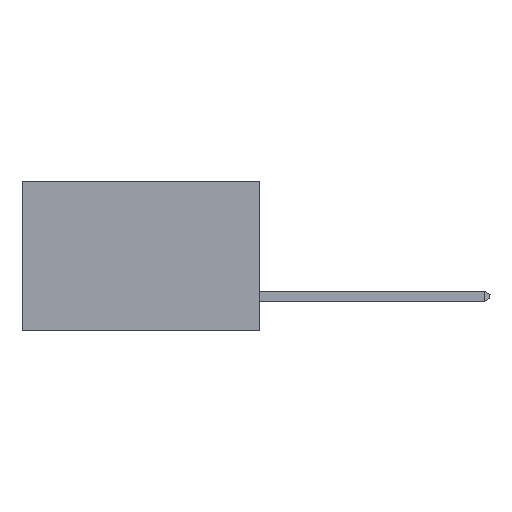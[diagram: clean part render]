
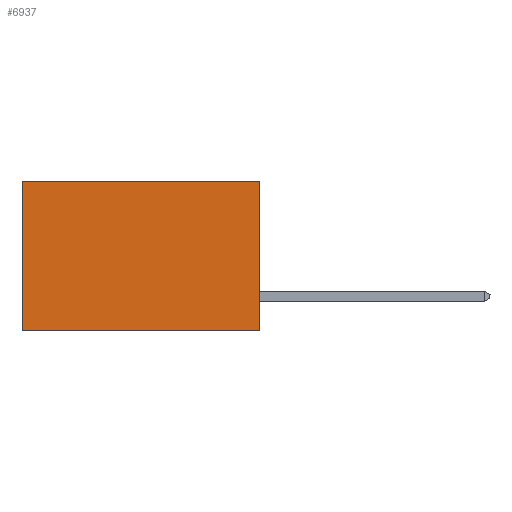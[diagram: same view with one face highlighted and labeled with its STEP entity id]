
A CAD part, left-side view. The second image highlights one B-rep face of the part: STEP entity #6937.
In plain terms, the highlighted planar face has unit normal (-1, 0, 0).
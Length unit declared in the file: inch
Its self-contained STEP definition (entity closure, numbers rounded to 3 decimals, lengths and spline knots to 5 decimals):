
#18 = FACE_OUTER_BOUND ( 'NONE', #20292, .T. ) ;
#437 = CARTESIAN_POINT ( 'NONE',  ( 0.277, 0., -0.37 ) ) ;
#490 = LINE ( 'NONE', #5966, #13847 ) ;
#847 = ORIENTED_EDGE ( 'NONE', *, *, #16687, .F. ) ;
#1221 = ORIENTED_EDGE ( 'NONE', *, *, #8267, .T. ) ;
#3124 = ORIENTED_EDGE ( 'NONE', *, *, #20080, .T. ) ;
#3379 = DIRECTION ( 'NONE',  ( 1., 0., 0. ) ) ;
#3512 = CARTESIAN_POINT ( 'NONE',  ( 0.277, 0., -0.37 ) ) ;
#4038 = AXIS2_PLACEMENT_3D ( 'NONE', #437, #3379, #16600 ) ;
#5423 = VERTEX_POINT ( 'NONE', #14707 ) ;
#5966 = CARTESIAN_POINT ( 'NONE',  ( 0.277, 0.59, -0.37 ) ) ;
#6185 = DIRECTION ( 'NONE',  ( 0., 0., -1. ) ) ;
#6362 = CARTESIAN_POINT ( 'NONE',  ( 0.277, 0.59, -0.37 ) ) ;
#6937 = ADVANCED_FACE ( 'NONE', ( #18 ), #7060, .F. ) ;
#7060 = PLANE ( 'NONE',  #4038 ) ;
#8267 = EDGE_CURVE ( 'NONE', #5423, #14977, #490, .T. ) ;
#8533 = VECTOR ( 'NONE', #20369, 39.37008 ) ;
#8921 = LINE ( 'NONE', #16401, #12975 ) ;
#9078 = LINE ( 'NONE', #3512, #8533 ) ;
#9322 = VECTOR ( 'NONE', #13610, 39.37008 ) ;
#9862 = LINE ( 'NONE', #16949, #9322 ) ;
#12975 = VECTOR ( 'NONE', #13107, 39.37008 ) ;
#13107 = DIRECTION ( 'NONE',  ( 0., 0., -1. ) ) ;
#13610 = DIRECTION ( 'NONE',  ( 0., 1., 0. ) ) ;
#13818 = CARTESIAN_POINT ( 'NONE',  ( 0.277, 0., -0.37 ) ) ;
#13847 = VECTOR ( 'NONE', #6185, 39.37008 ) ;
#13882 = ORIENTED_EDGE ( 'NONE', *, *, #19504, .F. ) ;
#14220 = CARTESIAN_POINT ( 'NONE',  ( 0.277, 0., 0. ) ) ;
#14707 = CARTESIAN_POINT ( 'NONE',  ( 0.277, 0.59, 0. ) ) ;
#14977 = VERTEX_POINT ( 'NONE', #6362 ) ;
#15650 = VERTEX_POINT ( 'NONE', #13818 ) ;
#16401 = CARTESIAN_POINT ( 'NONE',  ( 0.277, 0., -0.37 ) ) ;
#16600 = DIRECTION ( 'NONE',  ( 0., 0., -1. ) ) ;
#16687 = EDGE_CURVE ( 'NONE', #19612, #15650, #8921, .T. ) ;
#16949 = CARTESIAN_POINT ( 'NONE',  ( 0.277, 0., 0. ) ) ;
#19504 = EDGE_CURVE ( 'NONE', #15650, #14977, #9078, .T. ) ;
#19612 = VERTEX_POINT ( 'NONE', #14220 ) ;
#20080 = EDGE_CURVE ( 'NONE', #19612, #5423, #9862, .T. ) ;
#20292 = EDGE_LOOP ( 'NONE', ( #1221, #13882, #847, #3124 ) ) ;
#20369 = DIRECTION ( 'NONE',  ( 0., 1., 0. ) ) ;
